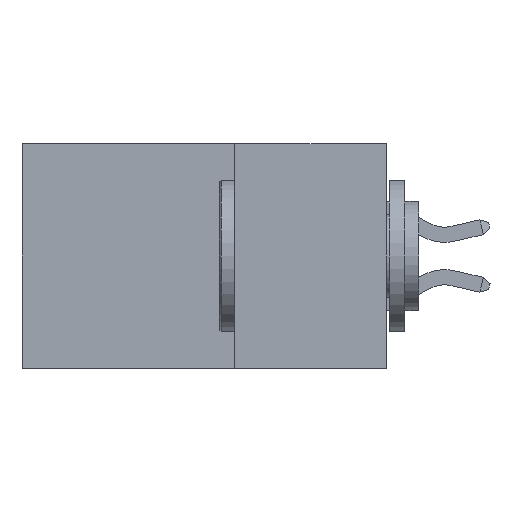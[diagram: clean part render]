
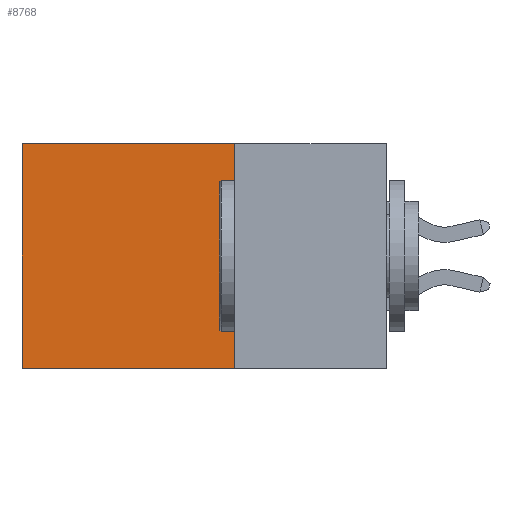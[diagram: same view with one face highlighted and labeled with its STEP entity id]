
A CAD part, left-side view. The second image highlights one B-rep face of the part: STEP entity #8768.
In plain terms, the highlighted planar face has unit normal (-1, 0, 0).
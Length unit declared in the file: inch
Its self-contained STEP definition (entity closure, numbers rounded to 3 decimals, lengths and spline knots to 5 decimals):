
#866 = VECTOR ( 'NONE', #10650, 39.37008 ) ;
#1000 = CARTESIAN_POINT ( 'NONE',  ( 0.298, 0.25, 0. ) ) ;
#1716 = ORIENTED_EDGE ( 'NONE', *, *, #3398, .T. ) ;
#2133 = VERTEX_POINT ( 'NONE', #1000 ) ;
#3398 = EDGE_CURVE ( 'NONE', #11521, #4716, #13692, .T. ) ;
#3557 = EDGE_CURVE ( 'NONE', #2133, #11521, #4598, .T. ) ;
#3841 = CARTESIAN_POINT ( 'NONE',  ( 0.298, 0.6, 0. ) ) ;
#4598 = LINE ( 'NONE', #7466, #8919 ) ;
#4716 = VERTEX_POINT ( 'NONE', #9971 ) ;
#4766 = CARTESIAN_POINT ( 'NONE',  ( 0.298, 0.25, -0.37 ) ) ;
#4855 = DIRECTION ( 'NONE',  ( 0., 1., 0. ) ) ;
#5538 = EDGE_CURVE ( 'NONE', #2133, #10016, #15596, .T. ) ;
#6005 = ORIENTED_EDGE ( 'NONE', *, *, #5538, .F. ) ;
#6620 = EDGE_CURVE ( 'NONE', #10016, #4716, #13447, .T. ) ;
#7377 = ORIENTED_EDGE ( 'NONE', *, *, #3557, .T. ) ;
#7466 = CARTESIAN_POINT ( 'NONE',  ( 0.298, 0.25, 0. ) ) ;
#8413 = CARTESIAN_POINT ( 'NONE',  ( 0.298, 0.6, 0. ) ) ;
#8427 = DIRECTION ( 'NONE',  ( 0., 0., -1. ) ) ;
#8714 = VECTOR ( 'NONE', #11174, 39.37008 ) ;
#8768 = ADVANCED_FACE ( 'NONE', ( #9721 ), #16856, .F. ) ;
#8919 = VECTOR ( 'NONE', #4855, 39.37008 ) ;
#9721 = FACE_OUTER_BOUND ( 'NONE', #16580, .T. ) ;
#9971 = CARTESIAN_POINT ( 'NONE',  ( 0.298, 0.6, -0.37 ) ) ;
#10016 = VERTEX_POINT ( 'NONE', #4766 ) ;
#10356 = CARTESIAN_POINT ( 'NONE',  ( 0.298, 0.25, 0. ) ) ;
#10650 = DIRECTION ( 'NONE',  ( 0., 0., -1. ) ) ;
#11174 = DIRECTION ( 'NONE',  ( 0., 0., -1. ) ) ;
#11521 = VERTEX_POINT ( 'NONE', #3841 ) ;
#11744 = ORIENTED_EDGE ( 'NONE', *, *, #6620, .F. ) ;
#12014 = AXIS2_PLACEMENT_3D ( 'NONE', #15373, #12512, #8427 ) ;
#12512 = DIRECTION ( 'NONE',  ( 1., 0., 0. ) ) ;
#13447 = LINE ( 'NONE', #16382, #17610 ) ;
#13692 = LINE ( 'NONE', #8413, #8714 ) ;
#15373 = CARTESIAN_POINT ( 'NONE',  ( 0.298, 0.25, 0. ) ) ;
#15596 = LINE ( 'NONE', #10356, #866 ) ;
#16382 = CARTESIAN_POINT ( 'NONE',  ( 0.298, 0.25, -0.37 ) ) ;
#16580 = EDGE_LOOP ( 'NONE', ( #1716, #11744, #6005, #7377 ) ) ;
#16856 = PLANE ( 'NONE',  #12014 ) ;
#17610 = VECTOR ( 'NONE', #17797, 39.37008 ) ;
#17797 = DIRECTION ( 'NONE',  ( 0., 1., 0. ) ) ;
